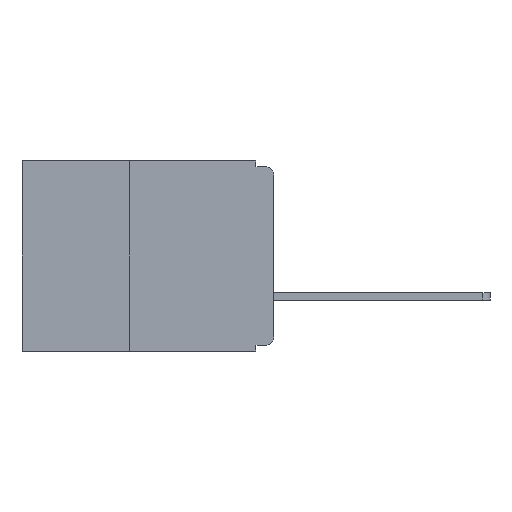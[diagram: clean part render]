
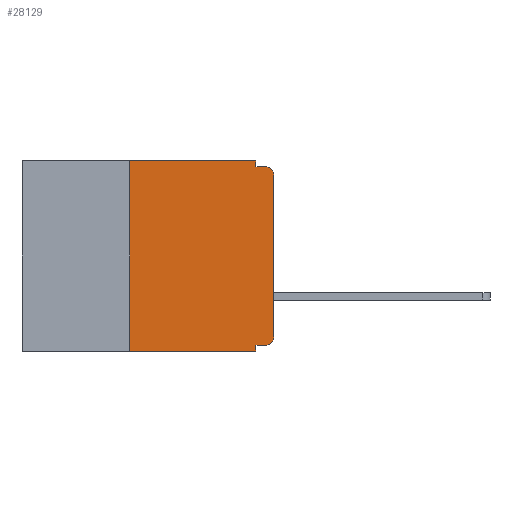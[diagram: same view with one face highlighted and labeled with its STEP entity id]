
A CAD part, left-side view. The second image highlights one B-rep face of the part: STEP entity #28129.
In plain terms, the highlighted planar face has unit normal (-1, 0, 0).
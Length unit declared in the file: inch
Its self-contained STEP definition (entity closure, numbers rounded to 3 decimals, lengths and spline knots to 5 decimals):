
#1032 = EDGE_LOOP ( 'NONE', ( #8031, #20433, #18632, #26203, #20798, #13558, #17230, #29398, #16977, #17472 ) ) ;
#1160 = FACE_OUTER_BOUND ( 'NONE', #1032, .T. ) ;
#1762 = VECTOR ( 'NONE', #6544, 39.37008 ) ;
#2456 = EDGE_CURVE ( 'NONE', #4252, #17297, #21820, .T. ) ;
#2906 = VERTEX_POINT ( 'NONE', #3785 ) ;
#3142 = CARTESIAN_POINT ( 'NONE',  ( 0., 0.25, -0.33 ) ) ;
#3764 = DIRECTION ( 'NONE',  ( 1., 0., 0. ) ) ;
#3785 = CARTESIAN_POINT ( 'NONE',  ( 0., 0.25, 0. ) ) ;
#4252 = VERTEX_POINT ( 'NONE', #21411 ) ;
#4494 = CARTESIAN_POINT ( 'NONE',  ( 0., 0.015, -0.025 ) ) ;
#4967 = CIRCLE ( 'NONE', #17588, 0.015 ) ;
#4997 = VECTOR ( 'NONE', #28008, 39.37008 ) ;
#5259 = DIRECTION ( 'NONE',  ( 0., -1., 0. ) ) ;
#5377 = VERTEX_POINT ( 'NONE', #5792 ) ;
#5509 = DIRECTION ( 'NONE',  ( 0., 0., 1. ) ) ;
#5548 = VERTEX_POINT ( 'NONE', #13454 ) ;
#5792 = CARTESIAN_POINT ( 'NONE',  ( 0., 0.031, -0.01 ) ) ;
#6245 = EDGE_CURVE ( 'NONE', #5377, #5548, #26518, .T. ) ;
#6544 = DIRECTION ( 'NONE',  ( 0., -1., 0. ) ) ;
#6824 = DIRECTION ( 'NONE',  ( 0., 0., -1. ) ) ;
#7009 = VECTOR ( 'NONE', #30058, 39.37008 ) ;
#7601 = CARTESIAN_POINT ( 'NONE',  ( 0., 0.031, 0. ) ) ;
#8031 = ORIENTED_EDGE ( 'NONE', *, *, #13317, .T. ) ;
#8767 = VERTEX_POINT ( 'NONE', #10322 ) ;
#9443 = VECTOR ( 'NONE', #27227, 39.37008 ) ;
#9842 = CARTESIAN_POINT ( 'NONE',  ( 0., 0.015, -0.305 ) ) ;
#10322 = CARTESIAN_POINT ( 'NONE',  ( 0., 0.25, -0.33 ) ) ;
#10489 = LINE ( 'NONE', #25752, #4997 ) ;
#10776 = LINE ( 'NONE', #3142, #28444 ) ;
#10988 = AXIS2_PLACEMENT_3D ( 'NONE', #9842, #26046, #12200 ) ;
#11055 = CARTESIAN_POINT ( 'NONE',  ( 0., 0., -0.305 ) ) ;
#11553 = VERTEX_POINT ( 'NONE', #11055 ) ;
#11824 = LINE ( 'NONE', #23248, #7009 ) ;
#11955 = CIRCLE ( 'NONE', #10988, 0.015 ) ;
#12092 = LINE ( 'NONE', #7601, #17548 ) ;
#12157 = CARTESIAN_POINT ( 'NONE',  ( 0., 0.031, -0.32 ) ) ;
#12200 = DIRECTION ( 'NONE',  ( 0., 0., -1. ) ) ;
#12333 = CARTESIAN_POINT ( 'NONE',  ( 0., 0.437, 0. ) ) ;
#13074 = PLANE ( 'NONE',  #22586 ) ;
#13157 = CARTESIAN_POINT ( 'NONE',  ( 0., 0., -0.32 ) ) ;
#13189 = DIRECTION ( 'NONE',  ( 0., 0., -1. ) ) ;
#13317 = EDGE_CURVE ( 'NONE', #11553, #21907, #10489, .T. ) ;
#13454 = CARTESIAN_POINT ( 'NONE',  ( 0., 0.015, -0.01 ) ) ;
#13492 = LINE ( 'NONE', #29142, #25093 ) ;
#13558 = ORIENTED_EDGE ( 'NONE', *, *, #20036, .F. ) ;
#13703 = EDGE_CURVE ( 'NONE', #21907, #5548, #4967, .T. ) ;
#14650 = DIRECTION ( 'NONE',  ( 0., 0., -1. ) ) ;
#15022 = EDGE_CURVE ( 'NONE', #8767, #27145, #11824, .T. ) ;
#16928 = EDGE_CURVE ( 'NONE', #17297, #27145, #13492, .T. ) ;
#16977 = ORIENTED_EDGE ( 'NONE', *, *, #2456, .F. ) ;
#17230 = ORIENTED_EDGE ( 'NONE', *, *, #15022, .T. ) ;
#17297 = VERTEX_POINT ( 'NONE', #12157 ) ;
#17472 = ORIENTED_EDGE ( 'NONE', *, *, #21780, .T. ) ;
#17548 = VECTOR ( 'NONE', #14650, 39.37008 ) ;
#17588 = AXIS2_PLACEMENT_3D ( 'NONE', #4494, #20788, #6824 ) ;
#18632 = ORIENTED_EDGE ( 'NONE', *, *, #6245, .F. ) ;
#19493 = LINE ( 'NONE', #12333, #24910 ) ;
#20036 = EDGE_CURVE ( 'NONE', #8767, #2906, #10776, .T. ) ;
#20070 = DIRECTION ( 'NONE',  ( 0., 0., -1. ) ) ;
#20433 = ORIENTED_EDGE ( 'NONE', *, *, #13703, .T. ) ;
#20788 = DIRECTION ( 'NONE',  ( -1., 0., 0. ) ) ;
#20798 = ORIENTED_EDGE ( 'NONE', *, *, #23072, .F. ) ;
#21411 = CARTESIAN_POINT ( 'NONE',  ( 0., 0.015, -0.32 ) ) ;
#21780 = EDGE_CURVE ( 'NONE', #4252, #11553, #11955, .T. ) ;
#21820 = LINE ( 'NONE', #13157, #9443 ) ;
#21836 = CARTESIAN_POINT ( 'NONE',  ( 0., 0., -0.025 ) ) ;
#21907 = VERTEX_POINT ( 'NONE', #21836 ) ;
#22586 = AXIS2_PLACEMENT_3D ( 'NONE', #28938, #3764, #20070 ) ;
#23072 = EDGE_CURVE ( 'NONE', #2906, #25506, #19493, .T. ) ;
#23143 = CARTESIAN_POINT ( 'NONE',  ( 0., 0.031, -0.33 ) ) ;
#23248 = CARTESIAN_POINT ( 'NONE',  ( 0., 0.437, -0.33 ) ) ;
#24910 = VECTOR ( 'NONE', #5259, 39.37008 ) ;
#25036 = EDGE_CURVE ( 'NONE', #25506, #5377, #12092, .T. ) ;
#25093 = VECTOR ( 'NONE', #13189, 39.37008 ) ;
#25506 = VERTEX_POINT ( 'NONE', #25649 ) ;
#25649 = CARTESIAN_POINT ( 'NONE',  ( 0., 0.031, 0. ) ) ;
#25752 = CARTESIAN_POINT ( 'NONE',  ( 0., 0., 0. ) ) ;
#26046 = DIRECTION ( 'NONE',  ( -1., 0., 0. ) ) ;
#26203 = ORIENTED_EDGE ( 'NONE', *, *, #25036, .F. ) ;
#26518 = LINE ( 'NONE', #29568, #1762 ) ;
#27145 = VERTEX_POINT ( 'NONE', #23143 ) ;
#27227 = DIRECTION ( 'NONE',  ( 0., 1., 0. ) ) ;
#28008 = DIRECTION ( 'NONE',  ( 0., 0., 1. ) ) ;
#28129 = ADVANCED_FACE ( 'NONE', ( #1160 ), #13074, .F. ) ;
#28444 = VECTOR ( 'NONE', #5509, 39.37008 ) ;
#28938 = CARTESIAN_POINT ( 'NONE',  ( 0., 0.437, 0. ) ) ;
#29142 = CARTESIAN_POINT ( 'NONE',  ( 0., 0.031, -0.33 ) ) ;
#29398 = ORIENTED_EDGE ( 'NONE', *, *, #16928, .F. ) ;
#29568 = CARTESIAN_POINT ( 'NONE',  ( 0., 0., -0.01 ) ) ;
#30058 = DIRECTION ( 'NONE',  ( 0., -1., 0. ) ) ;
